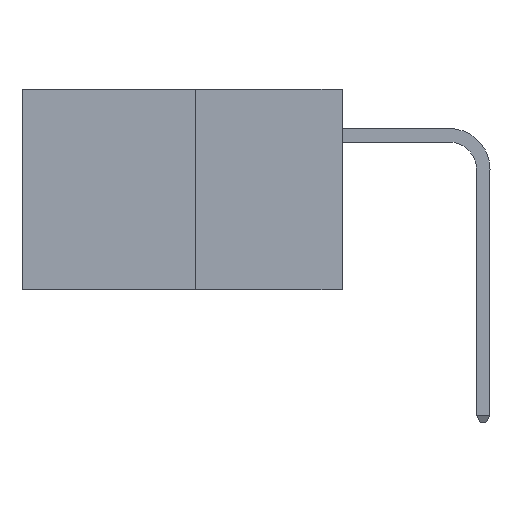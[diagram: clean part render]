
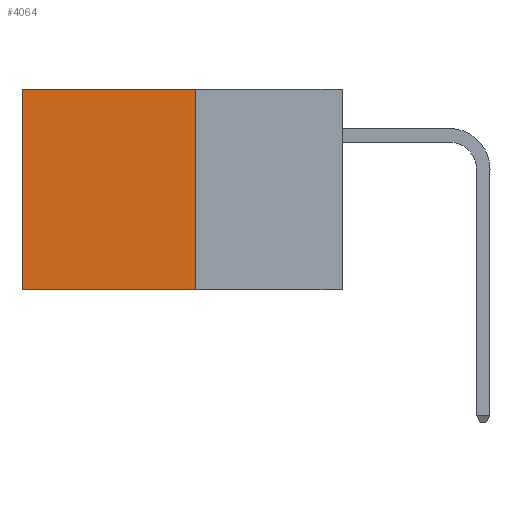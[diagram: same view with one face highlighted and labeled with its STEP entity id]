
A CAD part, left-side view. The second image highlights one B-rep face of the part: STEP entity #4064.
In plain terms, the highlighted planar face has unit normal (-1, 0, 0).
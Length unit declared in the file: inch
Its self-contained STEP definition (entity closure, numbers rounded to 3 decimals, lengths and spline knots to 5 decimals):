
#930 = EDGE_CURVE ( 'NONE', #9105, #3038, #9843, .T. ) ;
#1023 = DIRECTION ( 'NONE',  ( 0., 0., -1. ) ) ;
#1070 = DIRECTION ( 'NONE',  ( 0., 1., 0. ) ) ;
#1186 = EDGE_LOOP ( 'NONE', ( #4157, #5375, #9268, #6754 ) ) ;
#1212 = CARTESIAN_POINT ( 'NONE',  ( 0.277, 0.59, -0.37 ) ) ;
#1243 = CARTESIAN_POINT ( 'NONE',  ( 0.277, 0.27, -0.37 ) ) ;
#1284 = PLANE ( 'NONE',  #9249 ) ;
#2026 = CARTESIAN_POINT ( 'NONE',  ( 0.277, 0.27, -0.37 ) ) ;
#2184 = CARTESIAN_POINT ( 'NONE',  ( 0.277, 0.27, -0.37 ) ) ;
#2473 = CARTESIAN_POINT ( 'NONE',  ( 0.277, 0.27, -0.37 ) ) ;
#3038 = VERTEX_POINT ( 'NONE', #2184 ) ;
#3087 = EDGE_CURVE ( 'NONE', #9105, #5896, #7211, .T. ) ;
#3190 = VECTOR ( 'NONE', #1023, 39.37008 ) ;
#3508 = CARTESIAN_POINT ( 'NONE',  ( 0.277, 0.27, 0. ) ) ;
#4031 = VECTOR ( 'NONE', #9165, 39.37008 ) ;
#4064 = ADVANCED_FACE ( 'NONE', ( #5854 ), #1284, .F. ) ;
#4157 = ORIENTED_EDGE ( 'NONE', *, *, #7062, .T. ) ;
#4748 = DIRECTION ( 'NONE',  ( 1., 0., 0. ) ) ;
#5342 = EDGE_CURVE ( 'NONE', #3038, #10038, #6211, .T. ) ;
#5375 = ORIENTED_EDGE ( 'NONE', *, *, #5342, .F. ) ;
#5612 = DIRECTION ( 'NONE',  ( 0., 0., -1. ) ) ;
#5854 = FACE_OUTER_BOUND ( 'NONE', #1186, .T. ) ;
#5882 = CARTESIAN_POINT ( 'NONE',  ( 0.277, 0.27, 0. ) ) ;
#5896 = VERTEX_POINT ( 'NONE', #7335 ) ;
#6165 = DIRECTION ( 'NONE',  ( 0., 1., 0. ) ) ;
#6211 = LINE ( 'NONE', #1243, #6470 ) ;
#6449 = CARTESIAN_POINT ( 'NONE',  ( 0.277, 0.59, -0.37 ) ) ;
#6470 = VECTOR ( 'NONE', #1070, 39.37008 ) ;
#6754 = ORIENTED_EDGE ( 'NONE', *, *, #3087, .T. ) ;
#7062 = EDGE_CURVE ( 'NONE', #5896, #10038, #9085, .T. ) ;
#7211 = LINE ( 'NONE', #3508, #8905 ) ;
#7335 = CARTESIAN_POINT ( 'NONE',  ( 0.277, 0.59, 0. ) ) ;
#8905 = VECTOR ( 'NONE', #6165, 39.37008 ) ;
#9085 = LINE ( 'NONE', #1212, #3190 ) ;
#9105 = VERTEX_POINT ( 'NONE', #5882 ) ;
#9165 = DIRECTION ( 'NONE',  ( 0., 0., -1. ) ) ;
#9249 = AXIS2_PLACEMENT_3D ( 'NONE', #2026, #4748, #5612 ) ;
#9268 = ORIENTED_EDGE ( 'NONE', *, *, #930, .F. ) ;
#9843 = LINE ( 'NONE', #2473, #4031 ) ;
#10038 = VERTEX_POINT ( 'NONE', #6449 ) ;
